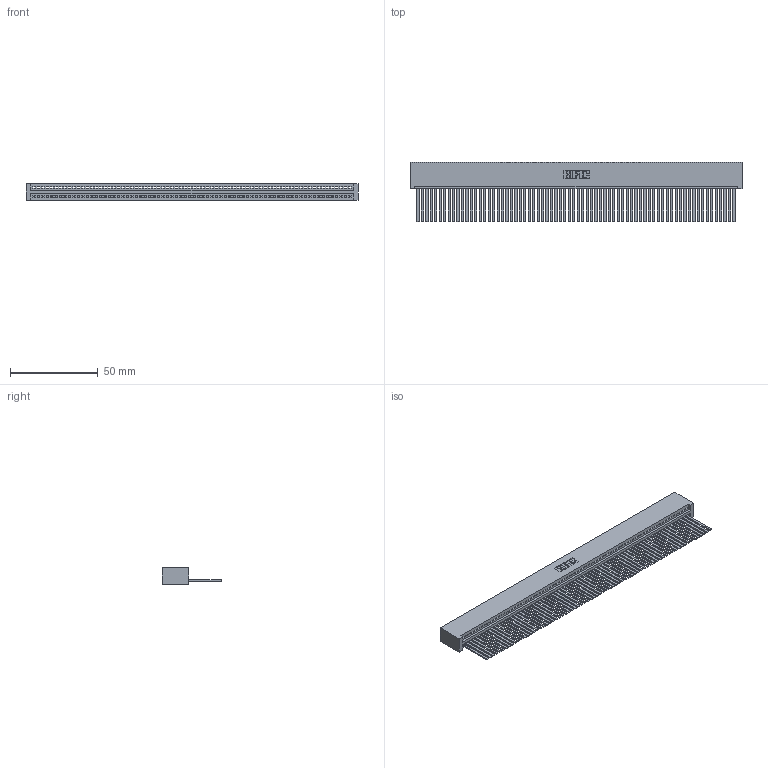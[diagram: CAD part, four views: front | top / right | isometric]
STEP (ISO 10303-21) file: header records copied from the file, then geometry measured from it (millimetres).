
FILE_DESCRIPTION (( 'STEP AP203' ), '1' );
FILE_NAME ('395-072-544-101.STEP', '2018-11-27T14:24:11', ( '' ), ( '' ), 'SwSTEP 2.0', 'SolidWorks 2016', '' );
FILE_SCHEMA (( 'CONFIG_CONTROL_DESIGN' ));
Length unit declared in the file: inch
Products named in the file (3): 345 Part_No Mounting Lugs; 395-072-544-101; 345-292-001_345-293-144
Assembly tree (73 placements, depth 2):
  395-072-544-101
    345 Part_No Mounting Lugs
    345-292-001_345-293-144  x72
Bounding box: 189.48 x 33.96 x 9.4 mm (x, y, z)
Volume: 19661.3 mm3; surface area: 29229.3 mm2
Topology: 73 solids, 73 shells, 3862 faces, 11693 edges, 7698 vertices
Faces by surface type: plane 2668, cylinder 1194
Entity records: 49689 total; most frequent: ORIENTED_EDGE 8618, CARTESIAN_POINT 8612, DIRECTION 7469, EDGE_CURVE 4309, LINE 3901, VECTOR 3901, VERTEX_POINT 2870, AXIS2_PLACEMENT_3D 1784
